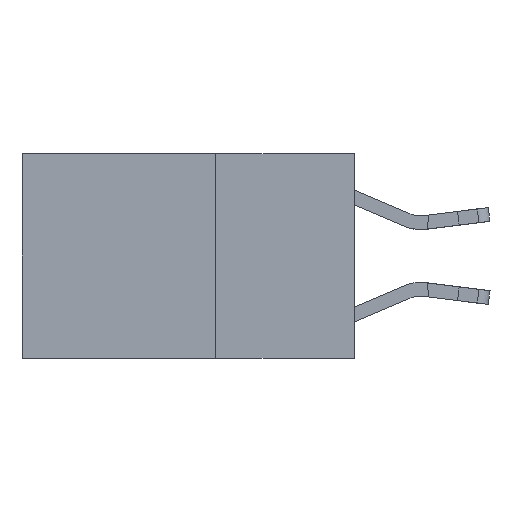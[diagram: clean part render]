
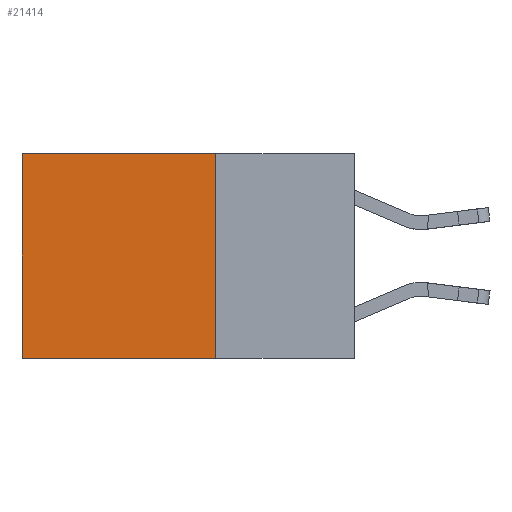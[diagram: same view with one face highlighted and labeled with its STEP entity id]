
A CAD part, left-side view. The second image highlights one B-rep face of the part: STEP entity #21414.
In plain terms, the highlighted planar face has unit normal (-1, 0, 0).
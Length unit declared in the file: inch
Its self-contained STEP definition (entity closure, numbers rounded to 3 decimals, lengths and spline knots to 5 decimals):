
#1155 = VECTOR ( 'NONE', #19554, 39.37008 ) ;
#2308 = CARTESIAN_POINT ( 'NONE',  ( 0.2625, 0.6, 0. ) ) ;
#2884 = VECTOR ( 'NONE', #7645, 39.37008 ) ;
#3729 = DIRECTION ( 'NONE',  ( 1., 0., 0. ) ) ;
#4069 = CARTESIAN_POINT ( 'NONE',  ( 0.2625, 0.25, -0.37 ) ) ;
#4089 = EDGE_CURVE ( 'NONE', #9484, #9968, #11657, .T. ) ;
#4873 = EDGE_LOOP ( 'NONE', ( #9180, #8375, #20567, #7454 ) ) ;
#5093 = EDGE_CURVE ( 'NONE', #9738, #9968, #10929, .T. ) ;
#7030 = CARTESIAN_POINT ( 'NONE',  ( 0.2625, 0.25, 0. ) ) ;
#7313 = CARTESIAN_POINT ( 'NONE',  ( 0.2625, 0.25, 0. ) ) ;
#7454 = ORIENTED_EDGE ( 'NONE', *, *, #8043, .T. ) ;
#7645 = DIRECTION ( 'NONE',  ( 0., 1., 0. ) ) ;
#8032 = CARTESIAN_POINT ( 'NONE',  ( 0.2625, 0.25, 0. ) ) ;
#8043 = EDGE_CURVE ( 'NONE', #11913, #9738, #21712, .T. ) ;
#8375 = ORIENTED_EDGE ( 'NONE', *, *, #4089, .F. ) ;
#8738 = DIRECTION ( 'NONE',  ( 0., 1., 0. ) ) ;
#8888 = CARTESIAN_POINT ( 'NONE',  ( 0.2625, 0.25, 0. ) ) ;
#9008 = EDGE_CURVE ( 'NONE', #11913, #9484, #13239, .T. ) ;
#9180 = ORIENTED_EDGE ( 'NONE', *, *, #5093, .T. ) ;
#9484 = VERTEX_POINT ( 'NONE', #11271 ) ;
#9738 = VERTEX_POINT ( 'NONE', #12627 ) ;
#9968 = VERTEX_POINT ( 'NONE', #16953 ) ;
#10698 = DIRECTION ( 'NONE',  ( 0., 0., -1. ) ) ;
#10929 = LINE ( 'NONE', #2308, #16116 ) ;
#11123 = DIRECTION ( 'NONE',  ( 0., 0., -1. ) ) ;
#11271 = CARTESIAN_POINT ( 'NONE',  ( 0.2625, 0.25, -0.37 ) ) ;
#11657 = LINE ( 'NONE', #4069, #2884 ) ;
#11913 = VERTEX_POINT ( 'NONE', #8032 ) ;
#12627 = CARTESIAN_POINT ( 'NONE',  ( 0.2625, 0.6, 0. ) ) ;
#13239 = LINE ( 'NONE', #7313, #1155 ) ;
#15043 = AXIS2_PLACEMENT_3D ( 'NONE', #7030, #3729, #10698 ) ;
#15421 = FACE_OUTER_BOUND ( 'NONE', #4873, .T. ) ;
#16027 = PLANE ( 'NONE',  #15043 ) ;
#16116 = VECTOR ( 'NONE', #11123, 39.37008 ) ;
#16953 = CARTESIAN_POINT ( 'NONE',  ( 0.2625, 0.6, -0.37 ) ) ;
#18698 = VECTOR ( 'NONE', #8738, 39.37008 ) ;
#19554 = DIRECTION ( 'NONE',  ( 0., 0., -1. ) ) ;
#20567 = ORIENTED_EDGE ( 'NONE', *, *, #9008, .F. ) ;
#21414 = ADVANCED_FACE ( 'NONE', ( #15421 ), #16027, .F. ) ;
#21712 = LINE ( 'NONE', #8888, #18698 ) ;
